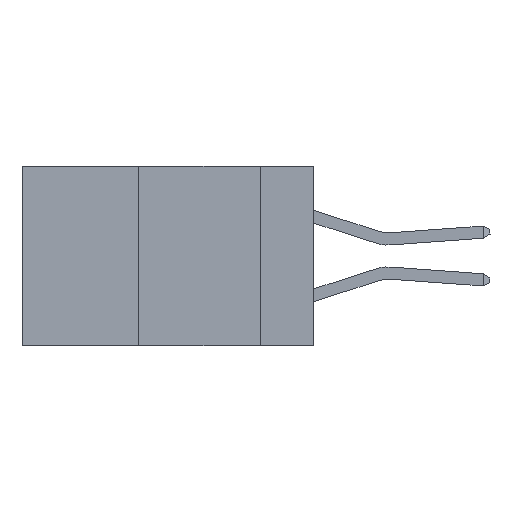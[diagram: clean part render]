
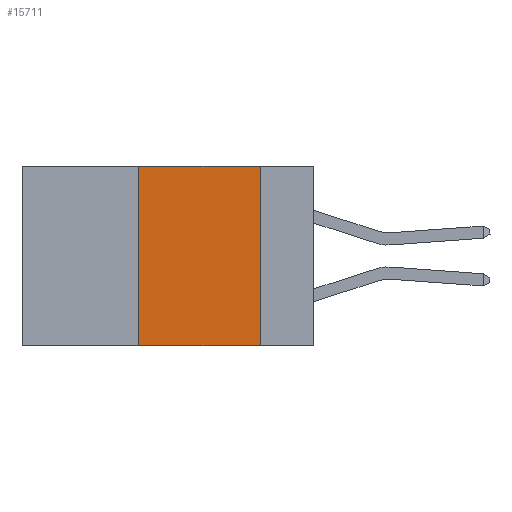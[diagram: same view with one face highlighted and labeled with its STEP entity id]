
A CAD part, left-side view. The second image highlights one B-rep face of the part: STEP entity #15711.
In plain terms, the highlighted planar face has unit normal (-1, 0, 0).
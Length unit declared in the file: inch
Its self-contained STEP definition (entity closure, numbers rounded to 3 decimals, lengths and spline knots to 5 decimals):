
#383 = LINE ( 'NONE', #11904, #5198 ) ;
#1458 = VECTOR ( 'NONE', #9886, 39.37008 ) ;
#1682 = CARTESIAN_POINT ( 'NONE',  ( 0., 0.6, -0.37 ) ) ;
#1827 = CARTESIAN_POINT ( 'NONE',  ( 0., 0.11, -0.37 ) ) ;
#2167 = CARTESIAN_POINT ( 'NONE',  ( 0., 0.6, 0. ) ) ;
#2236 = EDGE_CURVE ( 'NONE', #6595, #10016, #383, .T. ) ;
#2325 = ORIENTED_EDGE ( 'NONE', *, *, #8699, .F. ) ;
#2411 = VECTOR ( 'NONE', #15006, 39.37008 ) ;
#4737 = DIRECTION ( 'NONE',  ( 1., 0., 0. ) ) ;
#5160 = ORIENTED_EDGE ( 'NONE', *, *, #14235, .T. ) ;
#5198 = VECTOR ( 'NONE', #16237, 39.37008 ) ;
#5917 = EDGE_CURVE ( 'NONE', #11592, #15671, #15457, .T. ) ;
#6595 = VERTEX_POINT ( 'NONE', #6910 ) ;
#6644 = ORIENTED_EDGE ( 'NONE', *, *, #2236, .F. ) ;
#6910 = CARTESIAN_POINT ( 'NONE',  ( 0., 0.36, -0.37 ) ) ;
#7753 = PLANE ( 'NONE',  #10897 ) ;
#8699 = EDGE_CURVE ( 'NONE', #10016, #11592, #16697, .T. ) ;
#8839 = LINE ( 'NONE', #1682, #15089 ) ;
#9433 = CARTESIAN_POINT ( 'NONE',  ( 0., 0.36, 0. ) ) ;
#9886 = DIRECTION ( 'NONE',  ( 0., 0., -1. ) ) ;
#10016 = VERTEX_POINT ( 'NONE', #9433 ) ;
#10500 = DIRECTION ( 'NONE',  ( 0., 0., -1. ) ) ;
#10897 = AXIS2_PLACEMENT_3D ( 'NONE', #17685, #4737, #10500 ) ;
#11592 = VERTEX_POINT ( 'NONE', #14775 ) ;
#11771 = DIRECTION ( 'NONE',  ( 0., -1., 0. ) ) ;
#11904 = CARTESIAN_POINT ( 'NONE',  ( 0., 0.36, 0. ) ) ;
#12626 = CARTESIAN_POINT ( 'NONE',  ( 0., 0.11, 0. ) ) ;
#12889 = ORIENTED_EDGE ( 'NONE', *, *, #5917, .F. ) ;
#14235 = EDGE_CURVE ( 'NONE', #6595, #15671, #8839, .T. ) ;
#14654 = FACE_OUTER_BOUND ( 'NONE', #15128, .T. ) ;
#14775 = CARTESIAN_POINT ( 'NONE',  ( 0., 0.11, 0. ) ) ;
#15006 = DIRECTION ( 'NONE',  ( 0., -1., 0. ) ) ;
#15089 = VECTOR ( 'NONE', #11771, 39.37008 ) ;
#15128 = EDGE_LOOP ( 'NONE', ( #12889, #2325, #6644, #5160 ) ) ;
#15457 = LINE ( 'NONE', #12626, #1458 ) ;
#15671 = VERTEX_POINT ( 'NONE', #1827 ) ;
#15711 = ADVANCED_FACE ( 'NONE', ( #14654 ), #7753, .F. ) ;
#16237 = DIRECTION ( 'NONE',  ( 0., 0., 1. ) ) ;
#16697 = LINE ( 'NONE', #2167, #2411 ) ;
#17685 = CARTESIAN_POINT ( 'NONE',  ( 0., 0.6, 0. ) ) ;
